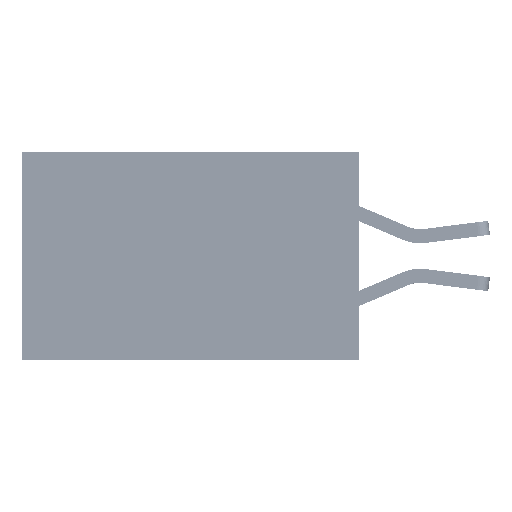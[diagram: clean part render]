
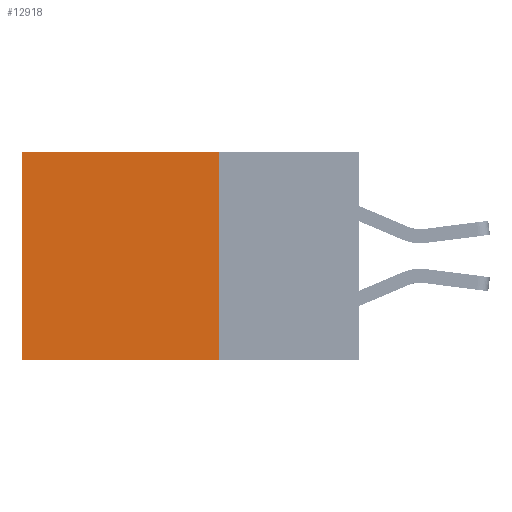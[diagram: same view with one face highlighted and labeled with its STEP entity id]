
A CAD part, left-side view. The second image highlights one B-rep face of the part: STEP entity #12918.
In plain terms, the highlighted planar face has unit normal (-1, 0, 0).
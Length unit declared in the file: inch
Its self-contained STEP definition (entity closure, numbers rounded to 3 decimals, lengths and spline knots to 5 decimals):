
#809 = VERTEX_POINT ( 'NONE', #39042 ) ;
#1627 = VERTEX_POINT ( 'NONE', #5476 ) ;
#2367 = FACE_OUTER_BOUND ( 'NONE', #19518, .T. ) ;
#3886 = DIRECTION ( 'NONE',  ( 0., 0., -1. ) ) ;
#5297 = EDGE_CURVE ( 'NONE', #1627, #809, #24559, .T. ) ;
#5476 = CARTESIAN_POINT ( 'NONE',  ( 0.2875, 0.6, 0. ) ) ;
#6877 = CARTESIAN_POINT ( 'NONE',  ( 0.2875, 0.25, -0.37 ) ) ;
#7363 = DIRECTION ( 'NONE',  ( 0., 1., 0. ) ) ;
#7617 = AXIS2_PLACEMENT_3D ( 'NONE', #15988, #12274, #12478 ) ;
#8766 = PLANE ( 'NONE',  #7617 ) ;
#9802 = ORIENTED_EDGE ( 'NONE', *, *, #15333, .F. ) ;
#12274 = DIRECTION ( 'NONE',  ( 1., 0., 0. ) ) ;
#12412 = ORIENTED_EDGE ( 'NONE', *, *, #30415, .F. ) ;
#12478 = DIRECTION ( 'NONE',  ( 0., 0., -1. ) ) ;
#12918 = ADVANCED_FACE ( 'NONE', ( #2367 ), #8766, .F. ) ;
#14587 = ORIENTED_EDGE ( 'NONE', *, *, #5297, .T. ) ;
#15333 = EDGE_CURVE ( 'NONE', #36699, #22429, #26218, .T. ) ;
#15988 = CARTESIAN_POINT ( 'NONE',  ( 0.2875, 0.25, 0. ) ) ;
#17605 = VECTOR ( 'NONE', #22405, 39.37008 ) ;
#18338 = DIRECTION ( 'NONE',  ( 0., 0., -1. ) ) ;
#19518 = EDGE_LOOP ( 'NONE', ( #14587, #12412, #9802, #22428 ) ) ;
#20529 = VECTOR ( 'NONE', #18338, 39.37008 ) ;
#21255 = CARTESIAN_POINT ( 'NONE',  ( 0.2875, 0.6, 0. ) ) ;
#21639 = CARTESIAN_POINT ( 'NONE',  ( 0.2875, 0.25, 0. ) ) ;
#22372 = EDGE_CURVE ( 'NONE', #36699, #1627, #40440, .T. ) ;
#22405 = DIRECTION ( 'NONE',  ( 0., 1., 0. ) ) ;
#22428 = ORIENTED_EDGE ( 'NONE', *, *, #22372, .T. ) ;
#22429 = VERTEX_POINT ( 'NONE', #6877 ) ;
#24559 = LINE ( 'NONE', #21255, #20529 ) ;
#25309 = CARTESIAN_POINT ( 'NONE',  ( 0.2875, 0.25, 0. ) ) ;
#26189 = LINE ( 'NONE', #35720, #38457 ) ;
#26218 = LINE ( 'NONE', #35136, #35281 ) ;
#30415 = EDGE_CURVE ( 'NONE', #22429, #809, #26189, .T. ) ;
#35136 = CARTESIAN_POINT ( 'NONE',  ( 0.2875, 0.25, 0. ) ) ;
#35281 = VECTOR ( 'NONE', #3886, 39.37008 ) ;
#35720 = CARTESIAN_POINT ( 'NONE',  ( 0.2875, 0.25, -0.37 ) ) ;
#36699 = VERTEX_POINT ( 'NONE', #21639 ) ;
#38457 = VECTOR ( 'NONE', #7363, 39.37008 ) ;
#39042 = CARTESIAN_POINT ( 'NONE',  ( 0.2875, 0.6, -0.37 ) ) ;
#40440 = LINE ( 'NONE', #25309, #17605 ) ;
